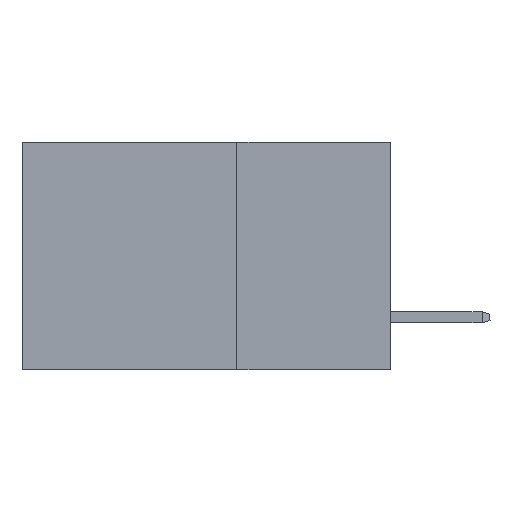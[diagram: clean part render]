
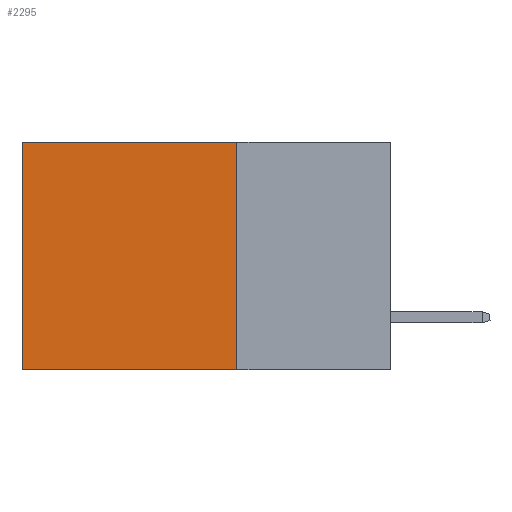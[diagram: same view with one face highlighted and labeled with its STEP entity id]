
A CAD part, left-side view. The second image highlights one B-rep face of the part: STEP entity #2295.
In plain terms, the highlighted planar face has unit normal (-1, 0, 0).
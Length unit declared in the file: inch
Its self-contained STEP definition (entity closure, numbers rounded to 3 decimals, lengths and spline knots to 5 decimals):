
#167 = CARTESIAN_POINT ( 'NONE',  ( 0.2875, 0.25, -0.37 ) ) ;
#1180 = CARTESIAN_POINT ( 'NONE',  ( 0.2875, 0.25, 0. ) ) ;
#1707 = CARTESIAN_POINT ( 'NONE',  ( 0.2875, 0.25, 0. ) ) ;
#2295 = ADVANCED_FACE ( 'NONE', ( #10320 ), #7935, .F. ) ;
#2673 = CARTESIAN_POINT ( 'NONE',  ( 0.2875, 0.6, -0.37 ) ) ;
#2785 = CARTESIAN_POINT ( 'NONE',  ( 0.2875, 0.25, -0.37 ) ) ;
#3054 = VECTOR ( 'NONE', #7222, 39.37008 ) ;
#3147 = VERTEX_POINT ( 'NONE', #2673 ) ;
#3745 = ORIENTED_EDGE ( 'NONE', *, *, #7992, .T. ) ;
#3980 = ORIENTED_EDGE ( 'NONE', *, *, #10737, .F. ) ;
#4113 = EDGE_LOOP ( 'NONE', ( #3745, #3980, #6486, #10536 ) ) ;
#4415 = VERTEX_POINT ( 'NONE', #2785 ) ;
#4792 = VECTOR ( 'NONE', #8597, 39.37008 ) ;
#5312 = AXIS2_PLACEMENT_3D ( 'NONE', #1180, #6524, #7979 ) ;
#5374 = CARTESIAN_POINT ( 'NONE',  ( 0.2875, 0.6, 0. ) ) ;
#5412 = CARTESIAN_POINT ( 'NONE',  ( 0.2875, 0.25, 0. ) ) ;
#5661 = LINE ( 'NONE', #10920, #3054 ) ;
#5712 = LINE ( 'NONE', #167, #7901 ) ;
#6486 = ORIENTED_EDGE ( 'NONE', *, *, #9158, .F. ) ;
#6524 = DIRECTION ( 'NONE',  ( 1., 0., 0. ) ) ;
#7222 = DIRECTION ( 'NONE',  ( 0., 0., -1. ) ) ;
#7268 = LINE ( 'NONE', #12220, #4792 ) ;
#7365 = LINE ( 'NONE', #1707, #11721 ) ;
#7629 = EDGE_CURVE ( 'NONE', #11376, #11727, #7268, .T. ) ;
#7901 = VECTOR ( 'NONE', #9951, 39.37008 ) ;
#7935 = PLANE ( 'NONE',  #5312 ) ;
#7979 = DIRECTION ( 'NONE',  ( 0., 0., -1. ) ) ;
#7992 = EDGE_CURVE ( 'NONE', #11727, #3147, #5661, .T. ) ;
#8509 = DIRECTION ( 'NONE',  ( 0., 0., -1. ) ) ;
#8597 = DIRECTION ( 'NONE',  ( 0., 1., 0. ) ) ;
#9158 = EDGE_CURVE ( 'NONE', #11376, #4415, #7365, .T. ) ;
#9951 = DIRECTION ( 'NONE',  ( 0., 1., 0. ) ) ;
#10320 = FACE_OUTER_BOUND ( 'NONE', #4113, .T. ) ;
#10536 = ORIENTED_EDGE ( 'NONE', *, *, #7629, .T. ) ;
#10737 = EDGE_CURVE ( 'NONE', #4415, #3147, #5712, .T. ) ;
#10920 = CARTESIAN_POINT ( 'NONE',  ( 0.2875, 0.6, 0. ) ) ;
#11376 = VERTEX_POINT ( 'NONE', #5412 ) ;
#11721 = VECTOR ( 'NONE', #8509, 39.37008 ) ;
#11727 = VERTEX_POINT ( 'NONE', #5374 ) ;
#12220 = CARTESIAN_POINT ( 'NONE',  ( 0.2875, 0.25, 0. ) ) ;
